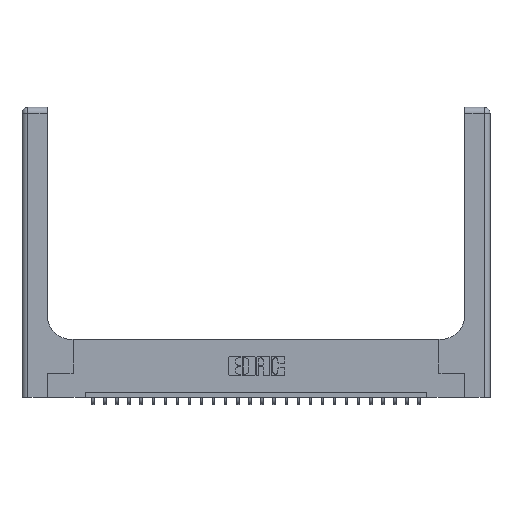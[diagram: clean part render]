
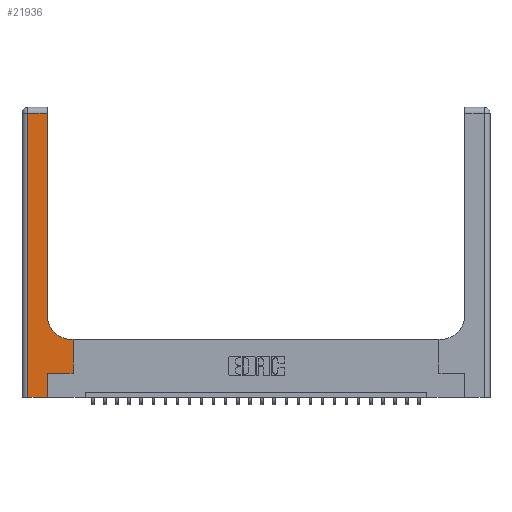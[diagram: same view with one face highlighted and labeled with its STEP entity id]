
A CAD part, top view. The second image highlights one B-rep face of the part: STEP entity #21936.
In plain terms, the highlighted planar face has unit normal (0, 0, 1).
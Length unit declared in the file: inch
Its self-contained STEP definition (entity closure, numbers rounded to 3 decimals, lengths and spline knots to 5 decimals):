
#162 = LINE ( 'NONE', #6144, #19208 ) ;
#873 = CARTESIAN_POINT ( 'NONE',  ( 0.528, 0.6, 0.37 ) ) ;
#889 = AXIS2_PLACEMENT_3D ( 'NONE', #21473, #10068, #23341 ) ;
#1154 = PLANE ( 'NONE',  #23406 ) ;
#1395 = CARTESIAN_POINT ( 'NONE',  ( 0., 0., 0.37 ) ) ;
#2210 = ORIENTED_EDGE ( 'NONE', *, *, #20524, .T. ) ;
#2516 = VERTEX_POINT ( 'NONE', #3724 ) ;
#3038 = DIRECTION ( 'NONE',  ( 0., 0., -1. ) ) ;
#3222 = LINE ( 'NONE', #6023, #22831 ) ;
#3375 = DIRECTION ( 'NONE',  ( 0., 1., 0. ) ) ;
#3388 = ORIENTED_EDGE ( 'NONE', *, *, #12411, .T. ) ;
#3606 = VECTOR ( 'NONE', #16615, 39.37008 ) ;
#3724 = CARTESIAN_POINT ( 'NONE',  ( 0.06, 2.94, 0.37 ) ) ;
#3879 = CARTESIAN_POINT ( 'NONE',  ( 0.265, 0.25, 0.37 ) ) ;
#3928 = CARTESIAN_POINT ( 'NONE',  ( 0.06, 3., 0.37 ) ) ;
#4294 = EDGE_CURVE ( 'NONE', #2516, #12638, #15966, .T. ) ;
#4332 = VERTEX_POINT ( 'NONE', #23019 ) ;
#4379 = CARTESIAN_POINT ( 'NONE',  ( 0.26, 0.85, 0.37 ) ) ;
#4950 = EDGE_CURVE ( 'NONE', #22454, #4332, #22428, .T. ) ;
#5723 = VERTEX_POINT ( 'NONE', #4379 ) ;
#6023 = CARTESIAN_POINT ( 'NONE',  ( 0.26, 3., 0.37 ) ) ;
#6061 = ORIENTED_EDGE ( 'NONE', *, *, #8155, .T. ) ;
#6144 = CARTESIAN_POINT ( 'NONE',  ( 0., 2.94, 0.37 ) ) ;
#6784 = VERTEX_POINT ( 'NONE', #8891 ) ;
#7420 = CARTESIAN_POINT ( 'NONE',  ( 0.265, 0.25, 0.37 ) ) ;
#7810 = DIRECTION ( 'NONE',  ( -1., 0., 0. ) ) ;
#8155 = EDGE_CURVE ( 'NONE', #6784, #11347, #19750, .T. ) ;
#8159 = LINE ( 'NONE', #24166, #17707 ) ;
#8217 = DIRECTION ( 'NONE',  ( -1., 0., 0. ) ) ;
#8460 = LINE ( 'NONE', #3879, #17416 ) ;
#8891 = CARTESIAN_POINT ( 'NONE',  ( 0.265, 0., 0.37 ) ) ;
#9580 = VECTOR ( 'NONE', #15264, 39.37008 ) ;
#10068 = DIRECTION ( 'NONE',  ( 0., 0., -1. ) ) ;
#11347 = VERTEX_POINT ( 'NONE', #7420 ) ;
#11893 = VERTEX_POINT ( 'NONE', #13153 ) ;
#12327 = EDGE_LOOP ( 'NONE', ( #12592, #23275, #19485, #24434, #6061, #2210, #12905, #18005, #3388 ) ) ;
#12411 = EDGE_CURVE ( 'NONE', #4332, #5723, #23333, .T. ) ;
#12592 = ORIENTED_EDGE ( 'NONE', *, *, #23607, .T. ) ;
#12638 = VERTEX_POINT ( 'NONE', #16405 ) ;
#12905 = ORIENTED_EDGE ( 'NONE', *, *, #13365, .T. ) ;
#13068 = EDGE_CURVE ( 'NONE', #17923, #2516, #162, .T. ) ;
#13153 = CARTESIAN_POINT ( 'NONE',  ( 0.528, 0.25, 0.37 ) ) ;
#13365 = EDGE_CURVE ( 'NONE', #11893, #22454, #8159, .T. ) ;
#13489 = CARTESIAN_POINT ( 'NONE',  ( 0.26, 0.6, 0.37 ) ) ;
#14934 = FACE_OUTER_BOUND ( 'NONE', #12327, .T. ) ;
#15177 = CARTESIAN_POINT ( 'NONE',  ( 0.265, 0., 0.37 ) ) ;
#15264 = DIRECTION ( 'NONE',  ( 0., 1., 0. ) ) ;
#15624 = DIRECTION ( 'NONE',  ( 0., 1., 0. ) ) ;
#15966 = LINE ( 'NONE', #3928, #20431 ) ;
#16359 = DIRECTION ( 'NONE',  ( -1., 0., 0. ) ) ;
#16405 = CARTESIAN_POINT ( 'NONE',  ( 0.06, 0., 0.37 ) ) ;
#16615 = DIRECTION ( 'NONE',  ( 1., 0., 0. ) ) ;
#17416 = VECTOR ( 'NONE', #22886, 39.37008 ) ;
#17707 = VECTOR ( 'NONE', #3375, 39.37008 ) ;
#17923 = VERTEX_POINT ( 'NONE', #22033 ) ;
#18005 = ORIENTED_EDGE ( 'NONE', *, *, #4950, .T. ) ;
#19178 = DIRECTION ( 'NONE',  ( 0., -1., 0. ) ) ;
#19208 = VECTOR ( 'NONE', #8217, 39.37008 ) ;
#19485 = ORIENTED_EDGE ( 'NONE', *, *, #4294, .T. ) ;
#19750 = LINE ( 'NONE', #15177, #9580 ) ;
#20109 = CARTESIAN_POINT ( 'NONE',  ( 0., 3., 0.37 ) ) ;
#20431 = VECTOR ( 'NONE', #19178, 39.37008 ) ;
#20524 = EDGE_CURVE ( 'NONE', #11347, #11893, #8460, .T. ) ;
#21473 = CARTESIAN_POINT ( 'NONE',  ( 0.51, 0.85, 0.37 ) ) ;
#21857 = VECTOR ( 'NONE', #7810, 39.37008 ) ;
#21936 = ADVANCED_FACE ( 'NONE', ( #14934 ), #1154, .F. ) ;
#22021 = EDGE_CURVE ( 'NONE', #12638, #6784, #23767, .T. ) ;
#22033 = CARTESIAN_POINT ( 'NONE',  ( 0.26, 2.94, 0.37 ) ) ;
#22428 = LINE ( 'NONE', #13489, #21857 ) ;
#22454 = VERTEX_POINT ( 'NONE', #873 ) ;
#22831 = VECTOR ( 'NONE', #15624, 39.37008 ) ;
#22886 = DIRECTION ( 'NONE',  ( 1., 0., 0. ) ) ;
#23019 = CARTESIAN_POINT ( 'NONE',  ( 0.51, 0.6, 0.37 ) ) ;
#23275 = ORIENTED_EDGE ( 'NONE', *, *, #13068, .T. ) ;
#23333 = CIRCLE ( 'NONE', #889, 0.25 ) ;
#23341 = DIRECTION ( 'NONE',  ( 1., 0., 0. ) ) ;
#23406 = AXIS2_PLACEMENT_3D ( 'NONE', #20109, #3038, #16359 ) ;
#23607 = EDGE_CURVE ( 'NONE', #5723, #17923, #3222, .T. ) ;
#23767 = LINE ( 'NONE', #1395, #3606 ) ;
#24166 = CARTESIAN_POINT ( 'NONE',  ( 0.528, 0.25, 0.37 ) ) ;
#24434 = ORIENTED_EDGE ( 'NONE', *, *, #22021, .T. ) ;
